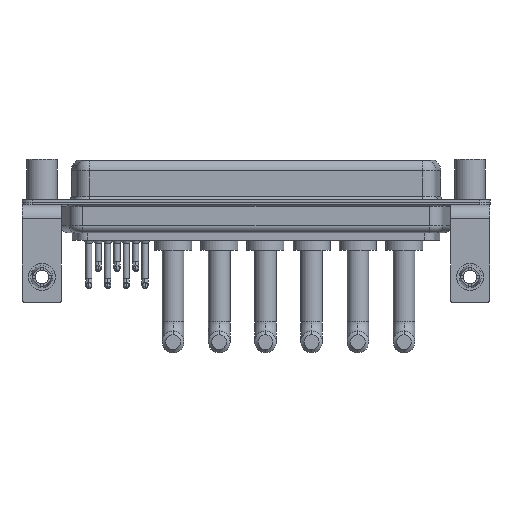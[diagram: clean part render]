
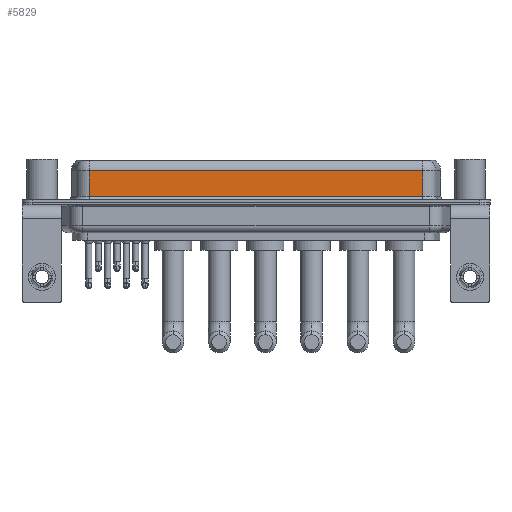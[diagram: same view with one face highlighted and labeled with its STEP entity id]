
A CAD part, front view. The second image highlights one B-rep face of the part: STEP entity #5829.
In plain terms, the highlighted planar face has unit normal (0, -1, 0).
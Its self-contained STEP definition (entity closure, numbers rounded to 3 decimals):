
#392 = EDGE_LOOP ( 'NONE', ( #1347, #7604, #11076, #2370 ) ) ;
#1212 = EDGE_CURVE ( 'NONE', #18449, #13778, #16911, .T. ) ;
#1347 = ORIENTED_EDGE ( 'NONE', *, *, #15292, .F. ) ;
#1527 = PLANE ( 'NONE',  #6808 ) ;
#1706 = CARTESIAN_POINT ( 'NONE',  ( 56.462, -3.95, 0.9 ) ) ;
#2198 = CARTESIAN_POINT ( 'NONE',  ( 7.038, -3.95, 0.9 ) ) ;
#2370 = ORIENTED_EDGE ( 'NONE', *, *, #4815, .T. ) ;
#2991 = DIRECTION ( 'NONE',  ( -1., 0., 0. ) ) ;
#2995 = DIRECTION ( 'NONE',  ( 0., 0., -1. ) ) ;
#3089 = CARTESIAN_POINT ( 'NONE',  ( 56.462, -3.95, 4.65 ) ) ;
#3194 = LINE ( 'NONE', #15422, #22221 ) ;
#3362 = FACE_OUTER_BOUND ( 'NONE', #392, .T. ) ;
#4289 = VECTOR ( 'NONE', #2991, 1000. ) ;
#4295 = EDGE_CURVE ( 'NONE', #13330, #18449, #22060, .T. ) ;
#4508 = VERTEX_POINT ( 'NONE', #1706 ) ;
#4799 = DIRECTION ( 'NONE',  ( 0., 0., -1. ) ) ;
#4815 = EDGE_CURVE ( 'NONE', #13778, #4508, #11639, .T. ) ;
#5664 = VECTOR ( 'NONE', #2995, 1000. ) ;
#5829 = ADVANCED_FACE ( 'NONE', ( #3362 ), #1527, .F. ) ;
#6287 = DIRECTION ( 'NONE',  ( 1., 0., 0. ) ) ;
#6808 = AXIS2_PLACEMENT_3D ( 'NONE', #10315, #17268, #13856 ) ;
#7604 = ORIENTED_EDGE ( 'NONE', *, *, #4295, .T. ) ;
#9600 = VECTOR ( 'NONE', #6287, 1000. ) ;
#9959 = CARTESIAN_POINT ( 'NONE',  ( 7.038, -3.95, 6.4 ) ) ;
#10315 = CARTESIAN_POINT ( 'NONE',  ( 56.462, -3.95, 6.4 ) ) ;
#11076 = ORIENTED_EDGE ( 'NONE', *, *, #1212, .T. ) ;
#11639 = LINE ( 'NONE', #13354, #9600 ) ;
#13330 = VERTEX_POINT ( 'NONE', #17420 ) ;
#13354 = CARTESIAN_POINT ( 'NONE',  ( 56.462, -3.95, 0.9 ) ) ;
#13778 = VERTEX_POINT ( 'NONE', #2198 ) ;
#13856 = DIRECTION ( 'NONE',  ( 0., 0., 1. ) ) ;
#15292 = EDGE_CURVE ( 'NONE', #13330, #4508, #3194, .T. ) ;
#15422 = CARTESIAN_POINT ( 'NONE',  ( 56.462, -3.95, 6.4 ) ) ;
#16911 = LINE ( 'NONE', #9959, #5664 ) ;
#17268 = DIRECTION ( 'NONE',  ( 0., 1., 0. ) ) ;
#17420 = CARTESIAN_POINT ( 'NONE',  ( 56.462, -3.95, 4.65 ) ) ;
#18449 = VERTEX_POINT ( 'NONE', #20077 ) ;
#20077 = CARTESIAN_POINT ( 'NONE',  ( 7.038, -3.95, 4.65 ) ) ;
#22060 = LINE ( 'NONE', #3089, #4289 ) ;
#22221 = VECTOR ( 'NONE', #4799, 1000. ) ;
